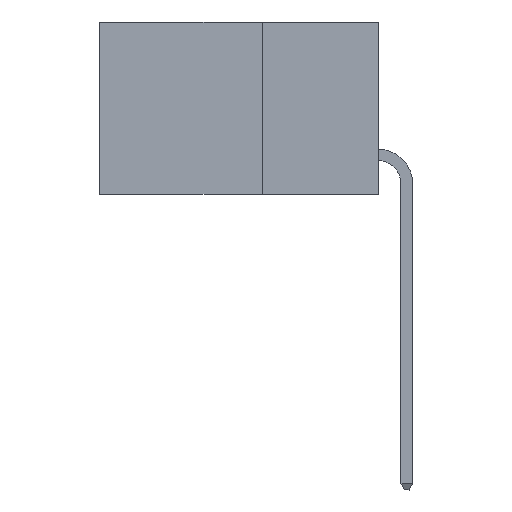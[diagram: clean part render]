
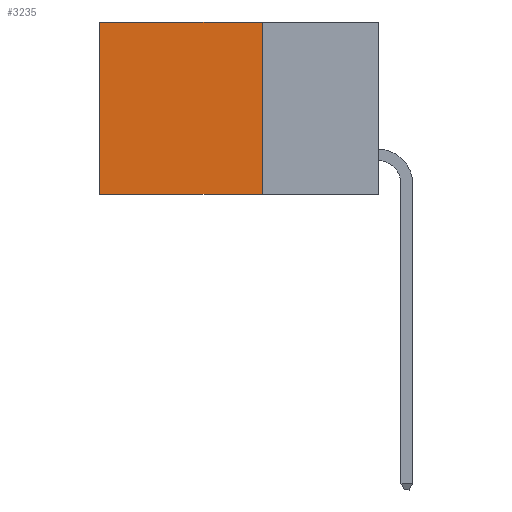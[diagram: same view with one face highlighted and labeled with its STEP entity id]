
A CAD part, left-side view. The second image highlights one B-rep face of the part: STEP entity #3235.
In plain terms, the highlighted planar face has unit normal (-1, 0, 0).
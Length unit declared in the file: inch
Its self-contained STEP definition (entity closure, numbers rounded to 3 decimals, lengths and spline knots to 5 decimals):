
#28 = VECTOR ( 'NONE', #13586, 39.37008 ) ;
#56 = EDGE_LOOP ( 'NONE', ( #11278, #11990, #6673, #3040 ) ) ;
#237 = VECTOR ( 'NONE', #8390, 39.37008 ) ;
#1187 = VECTOR ( 'NONE', #11155, 39.37008 ) ;
#1544 = LINE ( 'NONE', #2825, #237 ) ;
#2012 = FACE_OUTER_BOUND ( 'NONE', #56, .T. ) ;
#2387 = EDGE_CURVE ( 'NONE', #4483, #11118, #9179, .T. ) ;
#2825 = CARTESIAN_POINT ( 'NONE',  ( 0.2615, 0.25, -0.37 ) ) ;
#2951 = AXIS2_PLACEMENT_3D ( 'NONE', #6738, #6125, #5103 ) ;
#3040 = ORIENTED_EDGE ( 'NONE', *, *, #9610, .T. ) ;
#3235 = ADVANCED_FACE ( 'NONE', ( #2012 ), #12310, .F. ) ;
#3562 = CARTESIAN_POINT ( 'NONE',  ( 0.2615, 0.25, 0. ) ) ;
#3782 = CARTESIAN_POINT ( 'NONE',  ( 0.2615, 0.25, -0.37 ) ) ;
#4245 = VERTEX_POINT ( 'NONE', #13648 ) ;
#4483 = VERTEX_POINT ( 'NONE', #3562 ) ;
#5103 = DIRECTION ( 'NONE',  ( 0., 0., -1. ) ) ;
#6125 = DIRECTION ( 'NONE',  ( 1., 0., 0. ) ) ;
#6549 = VERTEX_POINT ( 'NONE', #6636 ) ;
#6636 = CARTESIAN_POINT ( 'NONE',  ( 0.2615, 0.6, -0.37 ) ) ;
#6673 = ORIENTED_EDGE ( 'NONE', *, *, #2387, .F. ) ;
#6738 = CARTESIAN_POINT ( 'NONE',  ( 0.2615, 0.25, -0.37 ) ) ;
#6776 = CARTESIAN_POINT ( 'NONE',  ( 0.2615, 0.6, -0.37 ) ) ;
#7563 = EDGE_CURVE ( 'NONE', #11118, #6549, #1544, .T. ) ;
#7989 = LINE ( 'NONE', #8071, #9631 ) ;
#8071 = CARTESIAN_POINT ( 'NONE',  ( 0.2615, 0.25, 0. ) ) ;
#8390 = DIRECTION ( 'NONE',  ( 0., 1., 0. ) ) ;
#9179 = LINE ( 'NONE', #3782, #28 ) ;
#9594 = LINE ( 'NONE', #6776, #1187 ) ;
#9610 = EDGE_CURVE ( 'NONE', #4483, #4245, #7989, .T. ) ;
#9631 = VECTOR ( 'NONE', #16399, 39.37008 ) ;
#11118 = VERTEX_POINT ( 'NONE', #13867 ) ;
#11155 = DIRECTION ( 'NONE',  ( 0., 0., -1. ) ) ;
#11278 = ORIENTED_EDGE ( 'NONE', *, *, #11976, .T. ) ;
#11976 = EDGE_CURVE ( 'NONE', #4245, #6549, #9594, .T. ) ;
#11990 = ORIENTED_EDGE ( 'NONE', *, *, #7563, .F. ) ;
#12310 = PLANE ( 'NONE',  #2951 ) ;
#13586 = DIRECTION ( 'NONE',  ( 0., 0., -1. ) ) ;
#13648 = CARTESIAN_POINT ( 'NONE',  ( 0.2615, 0.6, 0. ) ) ;
#13867 = CARTESIAN_POINT ( 'NONE',  ( 0.2615, 0.25, -0.37 ) ) ;
#16399 = DIRECTION ( 'NONE',  ( 0., 1., 0. ) ) ;
